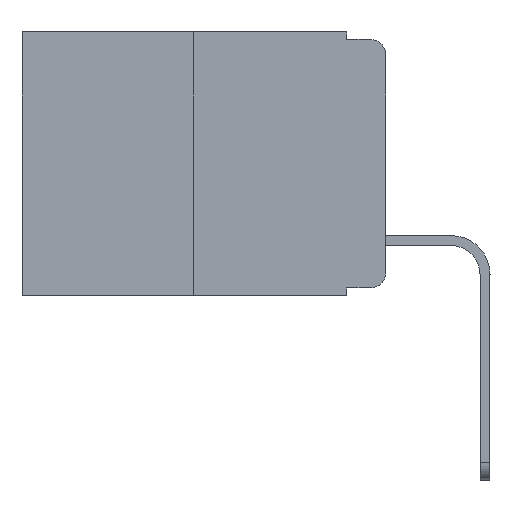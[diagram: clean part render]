
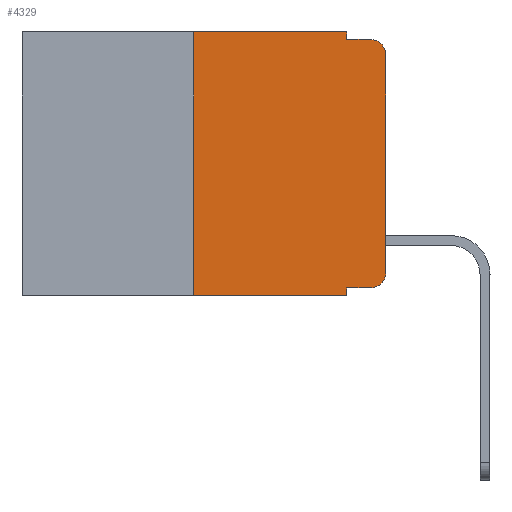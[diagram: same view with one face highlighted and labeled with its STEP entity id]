
A CAD part, left-side view. The second image highlights one B-rep face of the part: STEP entity #4329.
In plain terms, the highlighted planar face has unit normal (-1, 0, 0).
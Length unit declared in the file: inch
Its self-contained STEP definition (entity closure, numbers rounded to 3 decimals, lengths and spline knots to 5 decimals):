
#81 = CARTESIAN_POINT ( 'NONE',  ( 0., 0.25, 0. ) ) ;
#334 = ORIENTED_EDGE ( 'NONE', *, *, #7104, .T. ) ;
#354 = DIRECTION ( 'NONE',  ( -1., 0., 0. ) ) ;
#652 = LINE ( 'NONE', #7408, #8113 ) ;
#743 = VERTEX_POINT ( 'NONE', #9018 ) ;
#986 = ORIENTED_EDGE ( 'NONE', *, *, #12421, .F. ) ;
#1005 = AXIS2_PLACEMENT_3D ( 'NONE', #10764, #7864, #4645 ) ;
#1035 = CARTESIAN_POINT ( 'NONE',  ( 0., 0.473, -0.343 ) ) ;
#1052 = CARTESIAN_POINT ( 'NONE',  ( 0., 0.051, -0.01 ) ) ;
#1175 = DIRECTION ( 'NONE',  ( 0., 0., 1. ) ) ;
#1184 = DIRECTION ( 'NONE',  ( 0., 0., 1. ) ) ;
#1198 = LINE ( 'NONE', #8838, #3059 ) ;
#1340 = CARTESIAN_POINT ( 'NONE',  ( 0., 0.051, 0. ) ) ;
#1485 = EDGE_CURVE ( 'NONE', #7623, #6997, #12334, .T. ) ;
#1581 = DIRECTION ( 'NONE',  ( 0., 0., -1. ) ) ;
#2286 = ORIENTED_EDGE ( 'NONE', *, *, #13134, .F. ) ;
#2577 = CARTESIAN_POINT ( 'NONE',  ( 0., 0.02, -0.333 ) ) ;
#2653 = CARTESIAN_POINT ( 'NONE',  ( 0., 0.25, -0.343 ) ) ;
#2678 = VERTEX_POINT ( 'NONE', #12821 ) ;
#2718 = CARTESIAN_POINT ( 'NONE',  ( 0., 0.02, -0.01 ) ) ;
#2753 = ORIENTED_EDGE ( 'NONE', *, *, #9016, .T. ) ;
#2943 = ORIENTED_EDGE ( 'NONE', *, *, #13505, .F. ) ;
#3059 = VECTOR ( 'NONE', #9910, 39.37008 ) ;
#3072 = DIRECTION ( 'NONE',  ( 0., 0., -1. ) ) ;
#3090 = CARTESIAN_POINT ( 'NONE',  ( 0., 0., -0.03 ) ) ;
#3324 = CARTESIAN_POINT ( 'NONE',  ( 0., 0.051, -0.343 ) ) ;
#3589 = DIRECTION ( 'NONE',  ( 0., -1., 0. ) ) ;
#4222 = VECTOR ( 'NONE', #1184, 39.37008 ) ;
#4329 = ADVANCED_FACE ( 'NONE', ( #6721 ), #10991, .F. ) ;
#4438 = VERTEX_POINT ( 'NONE', #12331 ) ;
#4477 = CARTESIAN_POINT ( 'NONE',  ( 0., 0., 0. ) ) ;
#4645 = DIRECTION ( 'NONE',  ( 0., 0., -1. ) ) ;
#4723 = VECTOR ( 'NONE', #10994, 39.37008 ) ;
#4951 = LINE ( 'NONE', #4477, #11211 ) ;
#5063 = CARTESIAN_POINT ( 'NONE',  ( 0., 0.051, 0. ) ) ;
#5267 = VERTEX_POINT ( 'NONE', #3324 ) ;
#5401 = ORIENTED_EDGE ( 'NONE', *, *, #1485, .F. ) ;
#5549 = EDGE_CURVE ( 'NONE', #9149, #5267, #9875, .T. ) ;
#6251 = EDGE_LOOP ( 'NONE', ( #334, #2753, #986, #5401, #6463, #2286, #8625, #2943, #12005, #12348 ) ) ;
#6392 = CIRCLE ( 'NONE', #7038, 0.02 ) ;
#6463 = ORIENTED_EDGE ( 'NONE', *, *, #11928, .F. ) ;
#6721 = FACE_OUTER_BOUND ( 'NONE', #6251, .T. ) ;
#6874 = VECTOR ( 'NONE', #3589, 39.37008 ) ;
#6928 = LINE ( 'NONE', #12118, #4723 ) ;
#6997 = VERTEX_POINT ( 'NONE', #1052 ) ;
#7038 = AXIS2_PLACEMENT_3D ( 'NONE', #10237, #11388, #11246 ) ;
#7104 = EDGE_CURVE ( 'NONE', #4438, #8161, #4951, .T. ) ;
#7408 = CARTESIAN_POINT ( 'NONE',  ( 0., 0.051, 0. ) ) ;
#7623 = VERTEX_POINT ( 'NONE', #1340 ) ;
#7864 = DIRECTION ( 'NONE',  ( 1., 0., 0. ) ) ;
#7982 = CARTESIAN_POINT ( 'NONE',  ( 0., 0.02, -0.03 ) ) ;
#8113 = VECTOR ( 'NONE', #3072, 39.37008 ) ;
#8161 = VERTEX_POINT ( 'NONE', #3090 ) ;
#8625 = ORIENTED_EDGE ( 'NONE', *, *, #5549, .T. ) ;
#8838 = CARTESIAN_POINT ( 'NONE',  ( 0., 0.473, 0. ) ) ;
#9016 = EDGE_CURVE ( 'NONE', #8161, #12107, #11847, .T. ) ;
#9018 = CARTESIAN_POINT ( 'NONE',  ( 0., 0.051, -0.333 ) ) ;
#9073 = CARTESIAN_POINT ( 'NONE',  ( 0., 0.051, -0.333 ) ) ;
#9085 = EDGE_CURVE ( 'NONE', #10807, #4438, #6392, .T. ) ;
#9149 = VERTEX_POINT ( 'NONE', #2653 ) ;
#9437 = VECTOR ( 'NONE', #11454, 39.37008 ) ;
#9875 = LINE ( 'NONE', #1035, #10732 ) ;
#9910 = DIRECTION ( 'NONE',  ( 0., -1., 0. ) ) ;
#9979 = LINE ( 'NONE', #81, #4222 ) ;
#10237 = CARTESIAN_POINT ( 'NONE',  ( 0., 0.02, -0.313 ) ) ;
#10334 = EDGE_CURVE ( 'NONE', #743, #10807, #11099, .T. ) ;
#10732 = VECTOR ( 'NONE', #11692, 39.37008 ) ;
#10764 = CARTESIAN_POINT ( 'NONE',  ( 0., 0.473, 0. ) ) ;
#10807 = VERTEX_POINT ( 'NONE', #2577 ) ;
#10991 = PLANE ( 'NONE',  #1005 ) ;
#10994 = DIRECTION ( 'NONE',  ( 0., -1., 0. ) ) ;
#11099 = LINE ( 'NONE', #9073, #6874 ) ;
#11211 = VECTOR ( 'NONE', #1175, 39.37008 ) ;
#11246 = DIRECTION ( 'NONE',  ( 0., 0., -1. ) ) ;
#11388 = DIRECTION ( 'NONE',  ( -1., 0., 0. ) ) ;
#11454 = DIRECTION ( 'NONE',  ( 0., 0., -1. ) ) ;
#11692 = DIRECTION ( 'NONE',  ( 0., -1., 0. ) ) ;
#11847 = CIRCLE ( 'NONE', #12417, 0.02 ) ;
#11928 = EDGE_CURVE ( 'NONE', #2678, #7623, #1198, .T. ) ;
#12005 = ORIENTED_EDGE ( 'NONE', *, *, #10334, .T. ) ;
#12107 = VERTEX_POINT ( 'NONE', #2718 ) ;
#12118 = CARTESIAN_POINT ( 'NONE',  ( 0., 0.051, -0.01 ) ) ;
#12331 = CARTESIAN_POINT ( 'NONE',  ( 0., 0., -0.313 ) ) ;
#12334 = LINE ( 'NONE', #5063, #9437 ) ;
#12348 = ORIENTED_EDGE ( 'NONE', *, *, #9085, .T. ) ;
#12417 = AXIS2_PLACEMENT_3D ( 'NONE', #7982, #354, #1581 ) ;
#12421 = EDGE_CURVE ( 'NONE', #6997, #12107, #6928, .T. ) ;
#12821 = CARTESIAN_POINT ( 'NONE',  ( 0., 0.25, 0. ) ) ;
#13134 = EDGE_CURVE ( 'NONE', #9149, #2678, #9979, .T. ) ;
#13505 = EDGE_CURVE ( 'NONE', #743, #5267, #652, .T. ) ;
